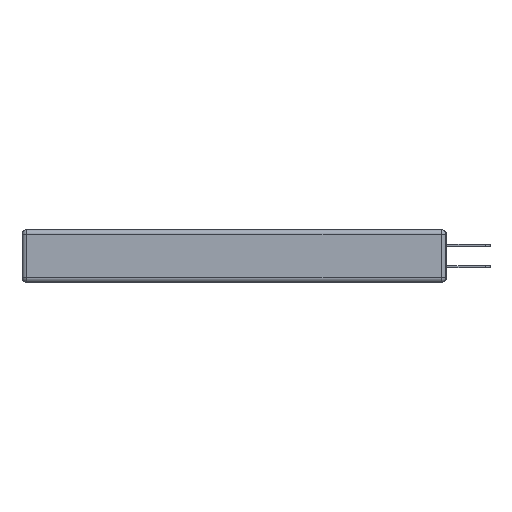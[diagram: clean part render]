
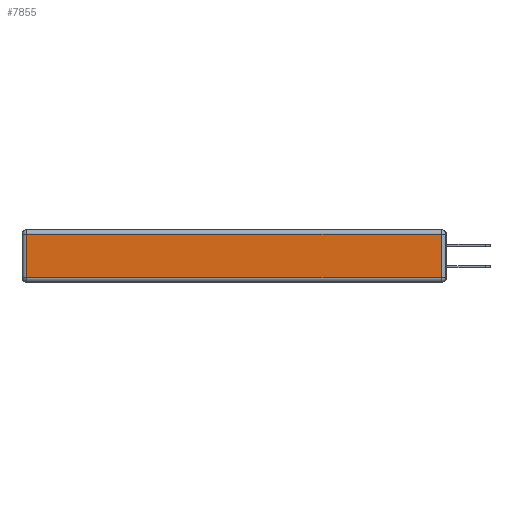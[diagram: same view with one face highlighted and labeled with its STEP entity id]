
A CAD part, left-side view. The second image highlights one B-rep face of the part: STEP entity #7855.
In plain terms, the highlighted planar face has unit normal (-1, 0, 0).
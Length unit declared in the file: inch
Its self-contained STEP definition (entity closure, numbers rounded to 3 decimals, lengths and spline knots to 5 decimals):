
#92 = VECTOR ( 'NONE', #14240, 39.37008 ) ;
#744 = VERTEX_POINT ( 'NONE', #1177 ) ;
#857 = EDGE_CURVE ( 'NONE', #3938, #17992, #8282, .T. ) ;
#1177 = CARTESIAN_POINT ( 'NONE',  ( 0., 0.03, -0.03 ) ) ;
#1265 = ORIENTED_EDGE ( 'NONE', *, *, #2162, .T. ) ;
#1490 = ORIENTED_EDGE ( 'NONE', *, *, #16570, .T. ) ;
#2162 = EDGE_CURVE ( 'NONE', #22132, #744, #18863, .T. ) ;
#2931 = DIRECTION ( 'NONE',  ( 0., -1., 0. ) ) ;
#3938 = VERTEX_POINT ( 'NONE', #13616 ) ;
#5916 = CARTESIAN_POINT ( 'NONE',  ( 0., 0., -0.343 ) ) ;
#6056 = DIRECTION ( 'NONE',  ( 0., 0., -1. ) ) ;
#6294 = DIRECTION ( 'NONE',  ( 0., 0., 1. ) ) ;
#6888 = CARTESIAN_POINT ( 'NONE',  ( 0., 0., -0.313 ) ) ;
#7855 = ADVANCED_FACE ( 'NONE', ( #19008 ), #19122, .T. ) ;
#8282 = LINE ( 'NONE', #9367, #21338 ) ;
#9367 = CARTESIAN_POINT ( 'NONE',  ( 0., 2.72, -0.343 ) ) ;
#10146 = AXIS2_PLACEMENT_3D ( 'NONE', #5916, #13476, #13388 ) ;
#11673 = EDGE_LOOP ( 'NONE', ( #22115, #1265, #1490, #18515 ) ) ;
#11953 = LINE ( 'NONE', #23896, #92 ) ;
#13388 = DIRECTION ( 'NONE',  ( 0., 0., 1. ) ) ;
#13476 = DIRECTION ( 'NONE',  ( -1., 0., 0. ) ) ;
#13616 = CARTESIAN_POINT ( 'NONE',  ( 0., 2.72, -0.03 ) ) ;
#14240 = DIRECTION ( 'NONE',  ( 0., 1., 0. ) ) ;
#14703 = CARTESIAN_POINT ( 'NONE',  ( 0., 0.03, -0.313 ) ) ;
#15493 = EDGE_CURVE ( 'NONE', #17992, #22132, #19603, .T. ) ;
#16142 = CARTESIAN_POINT ( 'NONE',  ( 0., 0.03, -0.343 ) ) ;
#16570 = EDGE_CURVE ( 'NONE', #744, #3938, #11953, .T. ) ;
#17992 = VERTEX_POINT ( 'NONE', #23837 ) ;
#18515 = ORIENTED_EDGE ( 'NONE', *, *, #857, .T. ) ;
#18863 = LINE ( 'NONE', #16142, #25214 ) ;
#19008 = FACE_OUTER_BOUND ( 'NONE', #11673, .T. ) ;
#19122 = PLANE ( 'NONE',  #10146 ) ;
#19603 = LINE ( 'NONE', #6888, #22902 ) ;
#21338 = VECTOR ( 'NONE', #6056, 39.37008 ) ;
#22115 = ORIENTED_EDGE ( 'NONE', *, *, #15493, .T. ) ;
#22132 = VERTEX_POINT ( 'NONE', #14703 ) ;
#22902 = VECTOR ( 'NONE', #2931, 39.37008 ) ;
#23837 = CARTESIAN_POINT ( 'NONE',  ( 0., 2.72, -0.313 ) ) ;
#23896 = CARTESIAN_POINT ( 'NONE',  ( 0., 2.75, -0.03 ) ) ;
#25214 = VECTOR ( 'NONE', #6294, 39.37008 ) ;
